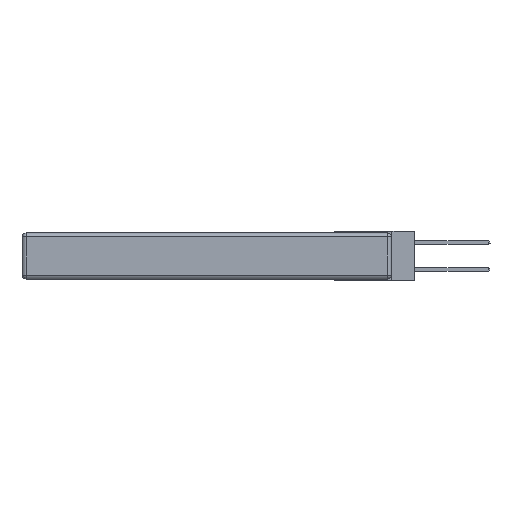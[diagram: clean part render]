
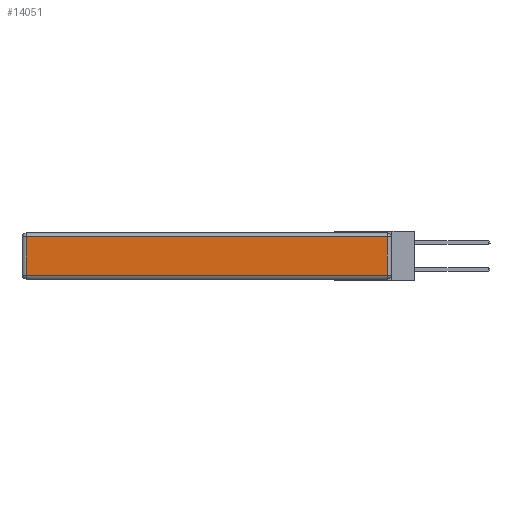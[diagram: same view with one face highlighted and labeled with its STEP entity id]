
A CAD part, left-side view. The second image highlights one B-rep face of the part: STEP entity #14051.
In plain terms, the highlighted planar face has unit normal (-1, 0, 0).
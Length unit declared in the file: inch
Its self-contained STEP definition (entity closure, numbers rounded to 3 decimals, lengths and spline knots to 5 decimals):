
#2 = EDGE_CURVE ( 'NONE', #6449, #2757, #17873, .T. ) ;
#209 = CARTESIAN_POINT ( 'NONE',  ( 0., 2.75, -0.03 ) ) ;
#2174 = LINE ( 'NONE', #17503, #16569 ) ;
#2549 = EDGE_CURVE ( 'NONE', #17020, #8468, #4876, .T. ) ;
#2757 = VERTEX_POINT ( 'NONE', #10875 ) ;
#2985 = DIRECTION ( 'NONE',  ( 0., 1., 0. ) ) ;
#3448 = EDGE_CURVE ( 'NONE', #8468, #6449, #16182, .T. ) ;
#3778 = ORIENTED_EDGE ( 'NONE', *, *, #12574, .T. ) ;
#4632 = VECTOR ( 'NONE', #15207, 39.37008 ) ;
#4876 = LINE ( 'NONE', #209, #14064 ) ;
#5110 = CARTESIAN_POINT ( 'NONE',  ( 0., 0., -0.313 ) ) ;
#5247 = ORIENTED_EDGE ( 'NONE', *, *, #2, .T. ) ;
#5666 = DIRECTION ( 'NONE',  ( -1., 0., 0. ) ) ;
#5694 = CARTESIAN_POINT ( 'NONE',  ( 0., 2.72, -0.03 ) ) ;
#6449 = VERTEX_POINT ( 'NONE', #11764 ) ;
#6476 = ORIENTED_EDGE ( 'NONE', *, *, #2549, .T. ) ;
#6495 = ORIENTED_EDGE ( 'NONE', *, *, #3448, .T. ) ;
#6526 = DIRECTION ( 'NONE',  ( 0., -1., 0. ) ) ;
#7794 = DIRECTION ( 'NONE',  ( 0., 0., 1. ) ) ;
#8468 = VERTEX_POINT ( 'NONE', #5694 ) ;
#10875 = CARTESIAN_POINT ( 'NONE',  ( 0., 0.03, -0.313 ) ) ;
#11764 = CARTESIAN_POINT ( 'NONE',  ( 0., 2.72, -0.313 ) ) ;
#12312 = AXIS2_PLACEMENT_3D ( 'NONE', #16672, #5666, #13884 ) ;
#12574 = EDGE_CURVE ( 'NONE', #2757, #17020, #2174, .T. ) ;
#13884 = DIRECTION ( 'NONE',  ( 0., 0., 1. ) ) ;
#14051 = ADVANCED_FACE ( 'NONE', ( #14333 ), #15217, .T. ) ;
#14064 = VECTOR ( 'NONE', #2985, 39.37008 ) ;
#14169 = VECTOR ( 'NONE', #6526, 39.37008 ) ;
#14333 = FACE_OUTER_BOUND ( 'NONE', #17915, .T. ) ;
#15207 = DIRECTION ( 'NONE',  ( 0., 0., -1. ) ) ;
#15217 = PLANE ( 'NONE',  #12312 ) ;
#16182 = LINE ( 'NONE', #16565, #4632 ) ;
#16565 = CARTESIAN_POINT ( 'NONE',  ( 0., 2.72, -0.343 ) ) ;
#16569 = VECTOR ( 'NONE', #7794, 39.37008 ) ;
#16672 = CARTESIAN_POINT ( 'NONE',  ( 0., 0., -0.343 ) ) ;
#16710 = CARTESIAN_POINT ( 'NONE',  ( 0., 0.03, -0.03 ) ) ;
#17020 = VERTEX_POINT ( 'NONE', #16710 ) ;
#17503 = CARTESIAN_POINT ( 'NONE',  ( 0., 0.03, -0.343 ) ) ;
#17873 = LINE ( 'NONE', #5110, #14169 ) ;
#17915 = EDGE_LOOP ( 'NONE', ( #5247, #3778, #6476, #6495 ) ) ;
